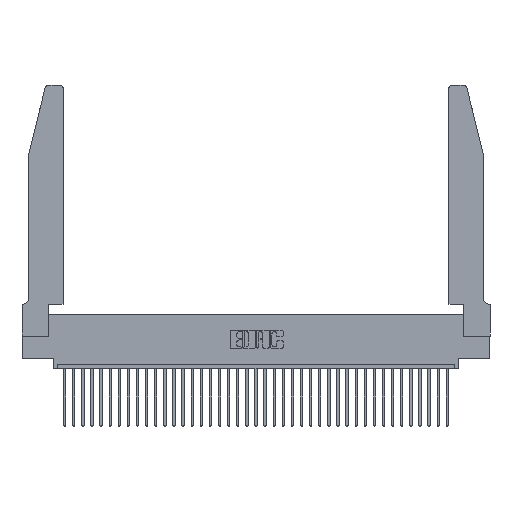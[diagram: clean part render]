
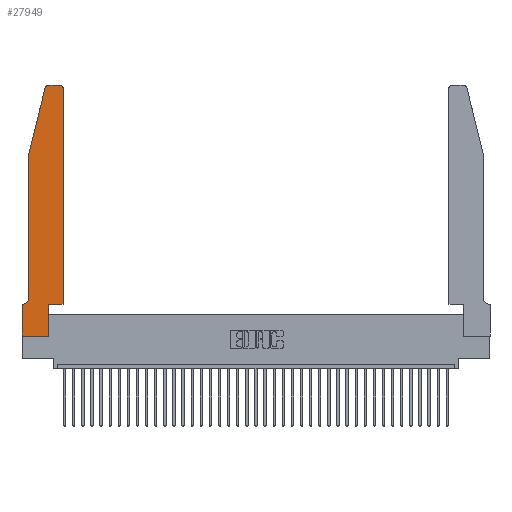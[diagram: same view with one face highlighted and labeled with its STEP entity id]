
A CAD part, top view. The second image highlights one B-rep face of the part: STEP entity #27949.
In plain terms, the highlighted planar face has unit normal (0, 0, 1).
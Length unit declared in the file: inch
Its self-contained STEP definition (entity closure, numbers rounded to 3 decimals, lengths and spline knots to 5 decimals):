
#315 = FACE_OUTER_BOUND ( 'NONE', #19705, .T. ) ;
#846 = ORIENTED_EDGE ( 'NONE', *, *, #2358, .T. ) ;
#978 = ORIENTED_EDGE ( 'NONE', *, *, #14774, .T. ) ;
#1077 = VECTOR ( 'NONE', #4705, 39.37008 ) ;
#1122 = CARTESIAN_POINT ( 'NONE',  ( 0.2865, 0., 0.37 ) ) ;
#1344 = CARTESIAN_POINT ( 'NONE',  ( 0.0755, 2., 0.37 ) ) ;
#2358 = EDGE_CURVE ( 'NONE', #4179, #30964, #15171, .T. ) ;
#2700 = CARTESIAN_POINT ( 'NONE',  ( 0.4205, 2.75, 0.37 ) ) ;
#2917 = VERTEX_POINT ( 'NONE', #11946 ) ;
#3115 = CARTESIAN_POINT ( 'NONE',  ( 0.0755, 2., 0.37 ) ) ;
#3514 = ORIENTED_EDGE ( 'NONE', *, *, #29928, .T. ) ;
#3681 = LINE ( 'NONE', #24670, #35056 ) ;
#4179 = VERTEX_POINT ( 'NONE', #5507 ) ;
#4705 = DIRECTION ( 'NONE',  ( -0.239, -0.971, 0. ) ) ;
#5313 = CARTESIAN_POINT ( 'NONE',  ( 0., 0., 0.37 ) ) ;
#5409 = VECTOR ( 'NONE', #34179, 39.37008 ) ;
#5505 = CARTESIAN_POINT ( 'NONE',  ( 0.4505, 0.35, 0.37 ) ) ;
#5507 = CARTESIAN_POINT ( 'NONE',  ( 0.0755, 0.42, 0.37 ) ) ;
#5826 = DIRECTION ( 'NONE',  ( 0., 0., -1. ) ) ;
#5952 = EDGE_CURVE ( 'NONE', #23193, #33824, #27387, .T. ) ;
#6151 = CIRCLE ( 'NONE', #31453, 0.03 ) ;
#6708 = ORIENTED_EDGE ( 'NONE', *, *, #8413, .T. ) ;
#6709 = LINE ( 'NONE', #24949, #24182 ) ;
#7429 = VECTOR ( 'NONE', #22262, 39.37008 ) ;
#7485 = ORIENTED_EDGE ( 'NONE', *, *, #22982, .T. ) ;
#7644 = LINE ( 'NONE', #26363, #16665 ) ;
#8413 = EDGE_CURVE ( 'NONE', #30964, #2917, #7644, .T. ) ;
#8716 = CARTESIAN_POINT ( 'NONE',  ( 0.25487, 2.72718, 0.37 ) ) ;
#10196 = DIRECTION ( 'NONE',  ( 0., 0., 1. ) ) ;
#10460 = ORIENTED_EDGE ( 'NONE', *, *, #34193, .T. ) ;
#10488 = CARTESIAN_POINT ( 'NONE',  ( 0.0755, 2., 0.37 ) ) ;
#10550 = DIRECTION ( 'NONE',  ( 1., 0., 0. ) ) ;
#10712 = DIRECTION ( 'NONE',  ( 0., 0., 1. ) ) ;
#11045 = DIRECTION ( 'NONE',  ( -1., 0., 0. ) ) ;
#11665 = VERTEX_POINT ( 'NONE', #33877 ) ;
#11825 = CARTESIAN_POINT ( 'NONE',  ( 0.4505, 2.72, 0.37 ) ) ;
#11831 = CARTESIAN_POINT ( 'NONE',  ( 0.2865, 0.35, 0.37 ) ) ;
#11946 = CARTESIAN_POINT ( 'NONE',  ( 0., 0.35, 0.37 ) ) ;
#12805 = AXIS2_PLACEMENT_3D ( 'NONE', #31126, #5826, #22528 ) ;
#13105 = DIRECTION ( 'NONE',  ( 0., 0., 1. ) ) ;
#13112 = LINE ( 'NONE', #28941, #35889 ) ;
#13151 = CARTESIAN_POINT ( 'NONE',  ( 0.4205, 2.72, 0.37 ) ) ;
#14294 = VECTOR ( 'NONE', #29176, 39.37008 ) ;
#14774 = EDGE_CURVE ( 'NONE', #33824, #16921, #22022, .T. ) ;
#15171 = CIRCLE ( 'NONE', #12805, 0.07 ) ;
#15626 = VERTEX_POINT ( 'NONE', #8716 ) ;
#16605 = DIRECTION ( 'NONE',  ( 1., 0., 0. ) ) ;
#16665 = VECTOR ( 'NONE', #17661, 39.37008 ) ;
#16921 = VERTEX_POINT ( 'NONE', #2700 ) ;
#17161 = EDGE_CURVE ( 'NONE', #28969, #15626, #6151, .T. ) ;
#17661 = DIRECTION ( 'NONE',  ( -1., 0., 0. ) ) ;
#18552 = ORIENTED_EDGE ( 'NONE', *, *, #33442, .T. ) ;
#19124 = CARTESIAN_POINT ( 'NONE',  ( 0., 0.35, 0.37 ) ) ;
#19705 = EDGE_LOOP ( 'NONE', ( #10460, #27249, #20293, #31233, #846, #6708, #3514, #7485, #31028, #18552, #21225, #978 ) ) ;
#20293 = ORIENTED_EDGE ( 'NONE', *, *, #30048, .T. ) ;
#20872 = CARTESIAN_POINT ( 'NONE',  ( 0.0055, 0.35, 0.37 ) ) ;
#21225 = ORIENTED_EDGE ( 'NONE', *, *, #5952, .T. ) ;
#22022 = CIRCLE ( 'NONE', #33818, 0.03 ) ;
#22262 = DIRECTION ( 'NONE',  ( 0., -1., 0. ) ) ;
#22370 = VERTEX_POINT ( 'NONE', #1344 ) ;
#22528 = DIRECTION ( 'NONE',  ( -1., 0., 0. ) ) ;
#22611 = LINE ( 'NONE', #11831, #25711 ) ;
#22875 = EDGE_CURVE ( 'NONE', #33572, #11665, #22611, .T. ) ;
#22982 = EDGE_CURVE ( 'NONE', #36450, #33572, #3681, .T. ) ;
#23193 = VERTEX_POINT ( 'NONE', #34335 ) ;
#24182 = VECTOR ( 'NONE', #11045, 39.37008 ) ;
#24242 = DIRECTION ( 'NONE',  ( 1., 0., 0. ) ) ;
#24604 = CARTESIAN_POINT ( 'NONE',  ( 0.284, 2.72, 0.37 ) ) ;
#24670 = CARTESIAN_POINT ( 'NONE',  ( 0., 0., 0.37 ) ) ;
#24945 = PLANE ( 'NONE',  #30584 ) ;
#24949 = CARTESIAN_POINT ( 'NONE',  ( 0.2605, 2.75, 0.37 ) ) ;
#25097 = DIRECTION ( 'NONE',  ( 1., 0., 0. ) ) ;
#25711 = VECTOR ( 'NONE', #35310, 39.37008 ) ;
#26187 = LINE ( 'NONE', #10488, #1077 ) ;
#26363 = CARTESIAN_POINT ( 'NONE',  ( 0.0755, 0.35, 0.37 ) ) ;
#27249 = ORIENTED_EDGE ( 'NONE', *, *, #17161, .T. ) ;
#27387 = LINE ( 'NONE', #5505, #5409 ) ;
#27949 = ADVANCED_FACE ( 'NONE', ( #315 ), #24945, .T. ) ;
#28941 = CARTESIAN_POINT ( 'NONE',  ( 0.4505, 0.35, 0.37 ) ) ;
#28969 = VERTEX_POINT ( 'NONE', #36627 ) ;
#29006 = EDGE_CURVE ( 'NONE', #22370, #4179, #37012, .T. ) ;
#29176 = DIRECTION ( 'NONE',  ( 0., -1., 0. ) ) ;
#29928 = EDGE_CURVE ( 'NONE', #2917, #36450, #34257, .T. ) ;
#30048 = EDGE_CURVE ( 'NONE', #15626, #22370, #26187, .T. ) ;
#30584 = AXIS2_PLACEMENT_3D ( 'NONE', #19124, #13105, #10550 ) ;
#30964 = VERTEX_POINT ( 'NONE', #20872 ) ;
#31028 = ORIENTED_EDGE ( 'NONE', *, *, #22875, .T. ) ;
#31126 = CARTESIAN_POINT ( 'NONE',  ( 0.0055, 0.42, 0.37 ) ) ;
#31233 = ORIENTED_EDGE ( 'NONE', *, *, #29006, .T. ) ;
#31335 = CARTESIAN_POINT ( 'NONE',  ( 0., 0., 0.37 ) ) ;
#31453 = AXIS2_PLACEMENT_3D ( 'NONE', #24604, #10712, #25097 ) ;
#32181 = DIRECTION ( 'NONE',  ( 1., 0., 0. ) ) ;
#33442 = EDGE_CURVE ( 'NONE', #11665, #23193, #13112, .T. ) ;
#33572 = VERTEX_POINT ( 'NONE', #1122 ) ;
#33818 = AXIS2_PLACEMENT_3D ( 'NONE', #13151, #10196, #24242 ) ;
#33824 = VERTEX_POINT ( 'NONE', #11825 ) ;
#33877 = CARTESIAN_POINT ( 'NONE',  ( 0.2865, 0.35, 0.37 ) ) ;
#34179 = DIRECTION ( 'NONE',  ( 0., 1., 0. ) ) ;
#34193 = EDGE_CURVE ( 'NONE', #16921, #28969, #6709, .T. ) ;
#34257 = LINE ( 'NONE', #5313, #7429 ) ;
#34335 = CARTESIAN_POINT ( 'NONE',  ( 0.4505, 0.35, 0.37 ) ) ;
#35056 = VECTOR ( 'NONE', #16605, 39.37008 ) ;
#35310 = DIRECTION ( 'NONE',  ( 0., 1., 0. ) ) ;
#35889 = VECTOR ( 'NONE', #32181, 39.37008 ) ;
#36450 = VERTEX_POINT ( 'NONE', #31335 ) ;
#36627 = CARTESIAN_POINT ( 'NONE',  ( 0.284, 2.75, 0.37 ) ) ;
#37012 = LINE ( 'NONE', #3115, #14294 ) ;
